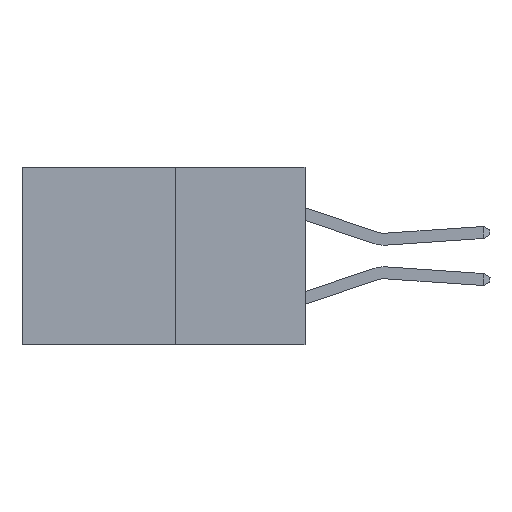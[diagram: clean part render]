
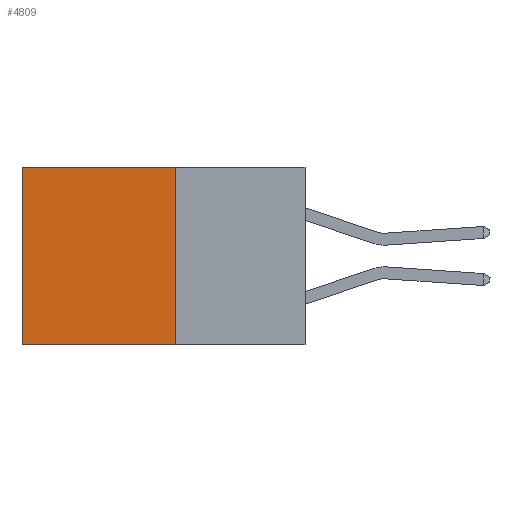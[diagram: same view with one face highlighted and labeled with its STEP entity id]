
A CAD part, left-side view. The second image highlights one B-rep face of the part: STEP entity #4809.
In plain terms, the highlighted planar face has unit normal (-1, 0, 0).
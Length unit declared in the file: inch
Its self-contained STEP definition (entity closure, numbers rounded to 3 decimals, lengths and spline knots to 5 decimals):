
#176 = CARTESIAN_POINT ( 'NONE',  ( 0.277, 0.59, -0.37 ) ) ;
#352 = CARTESIAN_POINT ( 'NONE',  ( 0.277, 0.59, 0. ) ) ;
#422 = LINE ( 'NONE', #5252, #5638 ) ;
#631 = LINE ( 'NONE', #3740, #2916 ) ;
#764 = DIRECTION ( 'NONE',  ( 0., 1., 0. ) ) ;
#916 = VECTOR ( 'NONE', #9031, 39.37008 ) ;
#1163 = PLANE ( 'NONE',  #8264 ) ;
#1340 = DIRECTION ( 'NONE',  ( 1., 0., 0. ) ) ;
#1434 = CARTESIAN_POINT ( 'NONE',  ( 0.277, 0.27, -0.37 ) ) ;
#1581 = ORIENTED_EDGE ( 'NONE', *, *, #8891, .T. ) ;
#1724 = DIRECTION ( 'NONE',  ( 0., 0., -1. ) ) ;
#2049 = EDGE_LOOP ( 'NONE', ( #1581, #7201, #8993, #7332 ) ) ;
#2233 = CARTESIAN_POINT ( 'NONE',  ( 0.277, 0.27, 0. ) ) ;
#2364 = VERTEX_POINT ( 'NONE', #4725 ) ;
#2916 = VECTOR ( 'NONE', #764, 39.37008 ) ;
#3740 = CARTESIAN_POINT ( 'NONE',  ( 0.277, 0.27, -0.37 ) ) ;
#4388 = DIRECTION ( 'NONE',  ( 0., 1., 0. ) ) ;
#4593 = EDGE_CURVE ( 'NONE', #5682, #2364, #422, .T. ) ;
#4714 = CARTESIAN_POINT ( 'NONE',  ( 0.277, 0.27, 0. ) ) ;
#4725 = CARTESIAN_POINT ( 'NONE',  ( 0.277, 0.27, -0.37 ) ) ;
#4809 = ADVANCED_FACE ( 'NONE', ( #10077 ), #1163, .F. ) ;
#5252 = CARTESIAN_POINT ( 'NONE',  ( 0.277, 0.27, -0.37 ) ) ;
#5638 = VECTOR ( 'NONE', #9881, 39.37008 ) ;
#5682 = VERTEX_POINT ( 'NONE', #2233 ) ;
#7201 = ORIENTED_EDGE ( 'NONE', *, *, #8439, .F. ) ;
#7249 = EDGE_CURVE ( 'NONE', #5682, #8862, #10299, .T. ) ;
#7332 = ORIENTED_EDGE ( 'NONE', *, *, #7249, .T. ) ;
#7953 = VECTOR ( 'NONE', #4388, 39.37008 ) ;
#8264 = AXIS2_PLACEMENT_3D ( 'NONE', #1434, #1340, #1724 ) ;
#8439 = EDGE_CURVE ( 'NONE', #2364, #9370, #631, .T. ) ;
#8862 = VERTEX_POINT ( 'NONE', #352 ) ;
#8891 = EDGE_CURVE ( 'NONE', #8862, #9370, #10657, .T. ) ;
#8993 = ORIENTED_EDGE ( 'NONE', *, *, #4593, .F. ) ;
#9031 = DIRECTION ( 'NONE',  ( 0., 0., -1. ) ) ;
#9370 = VERTEX_POINT ( 'NONE', #176 ) ;
#9881 = DIRECTION ( 'NONE',  ( 0., 0., -1. ) ) ;
#9889 = CARTESIAN_POINT ( 'NONE',  ( 0.277, 0.59, -0.37 ) ) ;
#10077 = FACE_OUTER_BOUND ( 'NONE', #2049, .T. ) ;
#10299 = LINE ( 'NONE', #4714, #7953 ) ;
#10657 = LINE ( 'NONE', #9889, #916 ) ;
